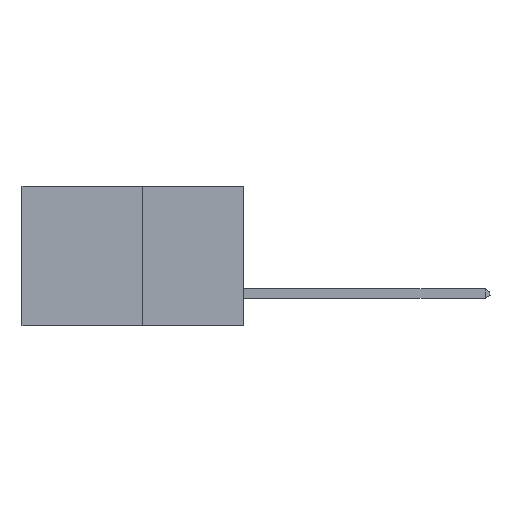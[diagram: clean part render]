
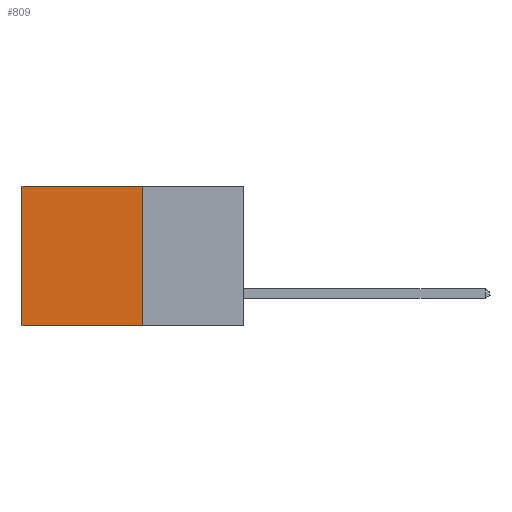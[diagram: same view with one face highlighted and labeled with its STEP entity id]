
A CAD part, left-side view. The second image highlights one B-rep face of the part: STEP entity #809.
In plain terms, the highlighted planar face has unit normal (-1, 0, 0).
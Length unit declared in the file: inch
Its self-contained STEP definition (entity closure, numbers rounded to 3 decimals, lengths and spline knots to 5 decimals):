
#64 = ORIENTED_EDGE ( 'NONE', *, *, #5529, .F. ) ;
#357 = DIRECTION ( 'NONE',  ( 1., 0., 0. ) ) ;
#452 = ORIENTED_EDGE ( 'NONE', *, *, #9982, .F. ) ;
#527 = CARTESIAN_POINT ( 'NONE',  ( 0.277, 0.27, 0. ) ) ;
#809 = ADVANCED_FACE ( 'NONE', ( #3785 ), #12085, .F. ) ;
#841 = EDGE_LOOP ( 'NONE', ( #12560, #452, #64, #3315 ) ) ;
#1062 = CARTESIAN_POINT ( 'NONE',  ( 0.277, 0.27, -0.37 ) ) ;
#1249 = DIRECTION ( 'NONE',  ( 0., 0., -1. ) ) ;
#1547 = LINE ( 'NONE', #4967, #7723 ) ;
#1677 = DIRECTION ( 'NONE',  ( 0., 1., 0. ) ) ;
#2837 = EDGE_CURVE ( 'NONE', #4421, #10893, #1547, .T. ) ;
#3315 = ORIENTED_EDGE ( 'NONE', *, *, #2837, .T. ) ;
#3785 = FACE_OUTER_BOUND ( 'NONE', #841, .T. ) ;
#4202 = VECTOR ( 'NONE', #7974, 39.37008 ) ;
#4248 = CARTESIAN_POINT ( 'NONE',  ( 0.277, 0.59, 0. ) ) ;
#4352 = VERTEX_POINT ( 'NONE', #1062 ) ;
#4421 = VERTEX_POINT ( 'NONE', #527 ) ;
#4563 = LINE ( 'NONE', #8079, #4202 ) ;
#4922 = DIRECTION ( 'NONE',  ( 0., 1., 0. ) ) ;
#4967 = CARTESIAN_POINT ( 'NONE',  ( 0.277, 0.27, 0. ) ) ;
#5529 = EDGE_CURVE ( 'NONE', #4421, #4352, #4563, .T. ) ;
#5961 = AXIS2_PLACEMENT_3D ( 'NONE', #8440, #357, #14749 ) ;
#7102 = CARTESIAN_POINT ( 'NONE',  ( 0.277, 0.59, -0.37 ) ) ;
#7723 = VECTOR ( 'NONE', #4922, 39.37008 ) ;
#7730 = EDGE_CURVE ( 'NONE', #10893, #12023, #8273, .T. ) ;
#7974 = DIRECTION ( 'NONE',  ( 0., 0., -1. ) ) ;
#8079 = CARTESIAN_POINT ( 'NONE',  ( 0.277, 0.27, -0.37 ) ) ;
#8273 = LINE ( 'NONE', #7102, #11357 ) ;
#8440 = CARTESIAN_POINT ( 'NONE',  ( 0.277, 0.27, -0.37 ) ) ;
#8608 = CARTESIAN_POINT ( 'NONE',  ( 0.277, 0.27, -0.37 ) ) ;
#8966 = VECTOR ( 'NONE', #1677, 39.37008 ) ;
#9982 = EDGE_CURVE ( 'NONE', #4352, #12023, #14763, .T. ) ;
#10893 = VERTEX_POINT ( 'NONE', #4248 ) ;
#11357 = VECTOR ( 'NONE', #1249, 39.37008 ) ;
#12023 = VERTEX_POINT ( 'NONE', #14305 ) ;
#12085 = PLANE ( 'NONE',  #5961 ) ;
#12560 = ORIENTED_EDGE ( 'NONE', *, *, #7730, .T. ) ;
#14305 = CARTESIAN_POINT ( 'NONE',  ( 0.277, 0.59, -0.37 ) ) ;
#14749 = DIRECTION ( 'NONE',  ( 0., 0., -1. ) ) ;
#14763 = LINE ( 'NONE', #8608, #8966 ) ;
